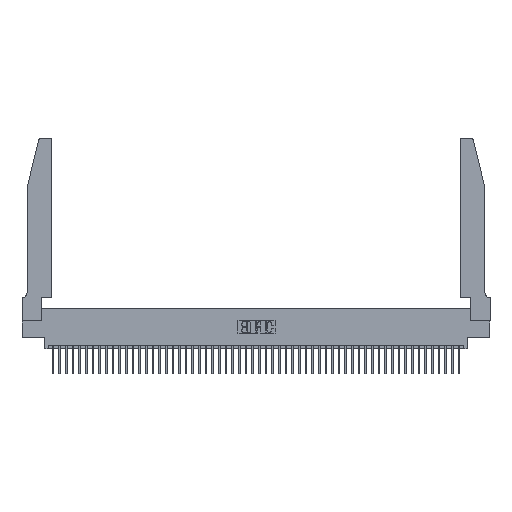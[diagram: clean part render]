
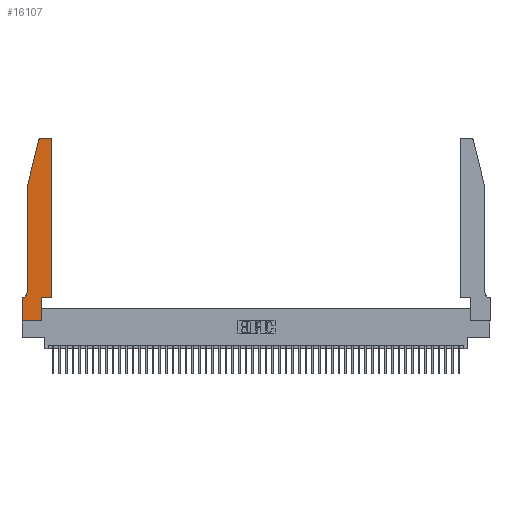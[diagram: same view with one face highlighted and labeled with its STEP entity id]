
A CAD part, top view. The second image highlights one B-rep face of the part: STEP entity #16107.
In plain terms, the highlighted planar face has unit normal (0, 0, 1).
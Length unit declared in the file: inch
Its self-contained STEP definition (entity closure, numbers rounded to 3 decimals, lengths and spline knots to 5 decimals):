
#86 = CARTESIAN_POINT ( 'NONE',  ( 0., 0., 0.37 ) ) ;
#113 = VERTEX_POINT ( 'NONE', #42085 ) ;
#296 = EDGE_CURVE ( 'NONE', #46229, #22425, #30796, .T. ) ;
#766 = CARTESIAN_POINT ( 'NONE',  ( 0.25487, 2.72718, 0.37 ) ) ;
#1017 = VERTEX_POINT ( 'NONE', #4301 ) ;
#1555 = EDGE_CURVE ( 'NONE', #46424, #113, #9762, .T. ) ;
#3104 = VECTOR ( 'NONE', #45747, 39.37008 ) ;
#3597 = DIRECTION ( 'NONE',  ( 0., 0., 1. ) ) ;
#4301 = CARTESIAN_POINT ( 'NONE',  ( 0.0055, 0.35, 0.37 ) ) ;
#6257 = CARTESIAN_POINT ( 'NONE',  ( 0.284, 2.72, 0.37 ) ) ;
#6596 = CARTESIAN_POINT ( 'NONE',  ( 0.0755, 2., 0.37 ) ) ;
#6619 = EDGE_CURVE ( 'NONE', #33950, #36148, #43828, .T. ) ;
#6733 = FACE_OUTER_BOUND ( 'NONE', #35941, .T. ) ;
#6773 = VERTEX_POINT ( 'NONE', #766 ) ;
#7692 = AXIS2_PLACEMENT_3D ( 'NONE', #43172, #24623, #27628 ) ;
#8102 = ORIENTED_EDGE ( 'NONE', *, *, #50393, .T. ) ;
#8163 = ORIENTED_EDGE ( 'NONE', *, *, #46537, .T. ) ;
#8186 = LINE ( 'NONE', #9795, #48684 ) ;
#8528 = VECTOR ( 'NONE', #18798, 39.37008 ) ;
#9094 = CARTESIAN_POINT ( 'NONE',  ( 0.4505, 0.35, 0.37 ) ) ;
#9282 = LINE ( 'NONE', #47149, #49759 ) ;
#9762 = LINE ( 'NONE', #26553, #8528 ) ;
#9795 = CARTESIAN_POINT ( 'NONE',  ( 0.4505, 0.35, 0.37 ) ) ;
#10242 = DIRECTION ( 'NONE',  ( 1., 0., 0. ) ) ;
#11471 = EDGE_CURVE ( 'NONE', #46604, #32611, #9282, .T. ) ;
#11796 = ORIENTED_EDGE ( 'NONE', *, *, #296, .T. ) ;
#11828 = LINE ( 'NONE', #49981, #31562 ) ;
#12035 = CARTESIAN_POINT ( 'NONE',  ( 0.0755, 2., 0.37 ) ) ;
#12312 = VECTOR ( 'NONE', #43246, 39.37008 ) ;
#15011 = VECTOR ( 'NONE', #31387, 39.37008 ) ;
#15104 = CARTESIAN_POINT ( 'NONE',  ( 0.2865, 0.35, 0.37 ) ) ;
#15481 = ORIENTED_EDGE ( 'NONE', *, *, #6619, .T. ) ;
#15810 = CARTESIAN_POINT ( 'NONE',  ( 0.0755, 2., 0.37 ) ) ;
#16107 = ADVANCED_FACE ( 'NONE', ( #6733 ), #35381, .T. ) ;
#16392 = CARTESIAN_POINT ( 'NONE',  ( 0.0755, 0.42, 0.37 ) ) ;
#16824 = DIRECTION ( 'NONE',  ( 0., 0., -1. ) ) ;
#17491 = VECTOR ( 'NONE', #33734, 39.37008 ) ;
#18798 = DIRECTION ( 'NONE',  ( -1., 0., 0. ) ) ;
#19241 = EDGE_CURVE ( 'NONE', #30490, #46604, #37335, .T. ) ;
#20554 = AXIS2_PLACEMENT_3D ( 'NONE', #27264, #3597, #31220 ) ;
#21323 = ORIENTED_EDGE ( 'NONE', *, *, #45445, .T. ) ;
#21351 = CARTESIAN_POINT ( 'NONE',  ( 0.4205, 2.75, 0.37 ) ) ;
#21475 = EDGE_CURVE ( 'NONE', #1017, #30490, #11828, .T. ) ;
#22385 = DIRECTION ( 'NONE',  ( 0., -1., 0. ) ) ;
#22425 = VERTEX_POINT ( 'NONE', #16392 ) ;
#22671 = AXIS2_PLACEMENT_3D ( 'NONE', #6257, #33881, #10242 ) ;
#24623 = DIRECTION ( 'NONE',  ( 0., 0., 1. ) ) ;
#25574 = CARTESIAN_POINT ( 'NONE',  ( 0.2865, 0., 0.37 ) ) ;
#26553 = CARTESIAN_POINT ( 'NONE',  ( 0.2605, 2.75, 0.37 ) ) ;
#26604 = CIRCLE ( 'NONE', #22671, 0.03 ) ;
#26871 = VECTOR ( 'NONE', #22385, 39.37008 ) ;
#27264 = CARTESIAN_POINT ( 'NONE',  ( 0.4205, 2.72, 0.37 ) ) ;
#27628 = DIRECTION ( 'NONE',  ( 1., 0., 0. ) ) ;
#27645 = CARTESIAN_POINT ( 'NONE',  ( 0.4505, 2.72, 0.37 ) ) ;
#27694 = DIRECTION ( 'NONE',  ( 1., 0., 0. ) ) ;
#27951 = LINE ( 'NONE', #41362, #17491 ) ;
#29490 = DIRECTION ( 'NONE',  ( 0., 1., 0. ) ) ;
#30490 = VERTEX_POINT ( 'NONE', #36710 ) ;
#30796 = LINE ( 'NONE', #15810, #12312 ) ;
#31220 = DIRECTION ( 'NONE',  ( 1., 0., 0. ) ) ;
#31387 = DIRECTION ( 'NONE',  ( 1., 0., 0. ) ) ;
#31562 = VECTOR ( 'NONE', #34564, 39.37008 ) ;
#32611 = VERTEX_POINT ( 'NONE', #25574 ) ;
#33377 = LINE ( 'NONE', #6596, #3104 ) ;
#33734 = DIRECTION ( 'NONE',  ( 0., 1., 0. ) ) ;
#33881 = DIRECTION ( 'NONE',  ( 0., 0., 1. ) ) ;
#33950 = VERTEX_POINT ( 'NONE', #15104 ) ;
#34090 = CARTESIAN_POINT ( 'NONE',  ( 0., 0., 0.37 ) ) ;
#34564 = DIRECTION ( 'NONE',  ( -1., 0., 0. ) ) ;
#34818 = CARTESIAN_POINT ( 'NONE',  ( 0.4505, 0.35, 0.37 ) ) ;
#35381 = PLANE ( 'NONE',  #7692 ) ;
#35941 = EDGE_LOOP ( 'NONE', ( #42672, #8102, #36400, #11796, #40707, #44088, #44525, #50569, #8163, #15481, #50509, #21323 ) ) ;
#36148 = VERTEX_POINT ( 'NONE', #9094 ) ;
#36400 = ORIENTED_EDGE ( 'NONE', *, *, #50457, .T. ) ;
#36710 = CARTESIAN_POINT ( 'NONE',  ( 0., 0.35, 0.37 ) ) ;
#37236 = CIRCLE ( 'NONE', #20554, 0.03 ) ;
#37335 = LINE ( 'NONE', #34090, #26871 ) ;
#37697 = CIRCLE ( 'NONE', #49788, 0.07 ) ;
#40354 = CARTESIAN_POINT ( 'NONE',  ( 0.0055, 0.42, 0.37 ) ) ;
#40707 = ORIENTED_EDGE ( 'NONE', *, *, #50168, .T. ) ;
#41362 = CARTESIAN_POINT ( 'NONE',  ( 0.2865, 0.35, 0.37 ) ) ;
#42085 = CARTESIAN_POINT ( 'NONE',  ( 0.284, 2.75, 0.37 ) ) ;
#42672 = ORIENTED_EDGE ( 'NONE', *, *, #1555, .T. ) ;
#43172 = CARTESIAN_POINT ( 'NONE',  ( 0., 0.35, 0.37 ) ) ;
#43246 = DIRECTION ( 'NONE',  ( 0., -1., 0. ) ) ;
#43828 = LINE ( 'NONE', #34818, #15011 ) ;
#44088 = ORIENTED_EDGE ( 'NONE', *, *, #21475, .T. ) ;
#44251 = DIRECTION ( 'NONE',  ( -1., 0., 0. ) ) ;
#44525 = ORIENTED_EDGE ( 'NONE', *, *, #19241, .T. ) ;
#44749 = VERTEX_POINT ( 'NONE', #27645 ) ;
#45445 = EDGE_CURVE ( 'NONE', #44749, #46424, #37236, .T. ) ;
#45747 = DIRECTION ( 'NONE',  ( -0.239, -0.971, 0. ) ) ;
#45837 = EDGE_CURVE ( 'NONE', #36148, #44749, #8186, .T. ) ;
#46229 = VERTEX_POINT ( 'NONE', #12035 ) ;
#46424 = VERTEX_POINT ( 'NONE', #21351 ) ;
#46537 = EDGE_CURVE ( 'NONE', #32611, #33950, #27951, .T. ) ;
#46604 = VERTEX_POINT ( 'NONE', #86 ) ;
#47149 = CARTESIAN_POINT ( 'NONE',  ( 0., 0., 0.37 ) ) ;
#48684 = VECTOR ( 'NONE', #29490, 39.37008 ) ;
#49759 = VECTOR ( 'NONE', #27694, 39.37008 ) ;
#49788 = AXIS2_PLACEMENT_3D ( 'NONE', #40354, #16824, #44251 ) ;
#49981 = CARTESIAN_POINT ( 'NONE',  ( 0.0755, 0.35, 0.37 ) ) ;
#50168 = EDGE_CURVE ( 'NONE', #22425, #1017, #37697, .T. ) ;
#50393 = EDGE_CURVE ( 'NONE', #113, #6773, #26604, .T. ) ;
#50457 = EDGE_CURVE ( 'NONE', #6773, #46229, #33377, .T. ) ;
#50509 = ORIENTED_EDGE ( 'NONE', *, *, #45837, .T. ) ;
#50569 = ORIENTED_EDGE ( 'NONE', *, *, #11471, .T. ) ;
